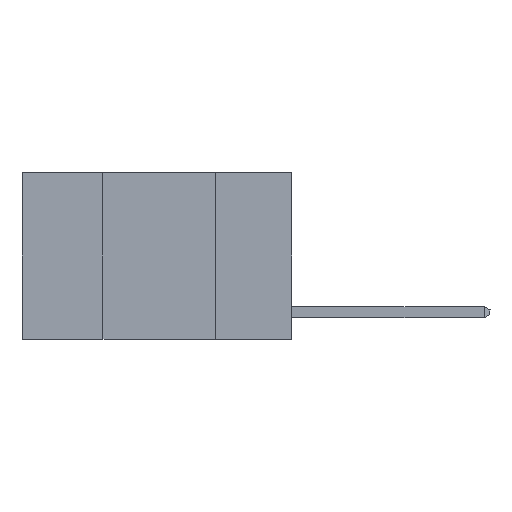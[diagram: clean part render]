
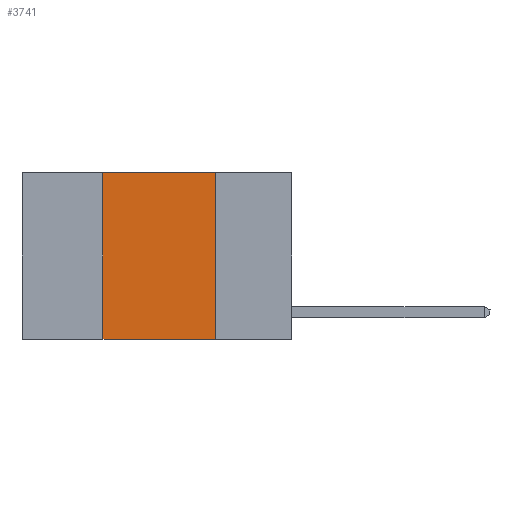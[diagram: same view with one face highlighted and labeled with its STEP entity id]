
A CAD part, left-side view. The second image highlights one B-rep face of the part: STEP entity #3741.
In plain terms, the highlighted planar face has unit normal (-1, 0, 0).
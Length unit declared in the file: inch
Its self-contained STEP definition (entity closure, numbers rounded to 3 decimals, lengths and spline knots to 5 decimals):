
#1185 = CARTESIAN_POINT ( 'NONE',  ( 0., 0.17, 0. ) ) ;
#2030 = ORIENTED_EDGE ( 'NONE', *, *, #6733, .F. ) ;
#2066 = LINE ( 'NONE', #9110, #14103 ) ;
#2395 = CARTESIAN_POINT ( 'NONE',  ( 0., 0.6, -0.37 ) ) ;
#2451 = DIRECTION ( 'NONE',  ( 0., 0., 1. ) ) ;
#3520 = PLANE ( 'NONE',  #16360 ) ;
#3563 = EDGE_CURVE ( 'NONE', #4761, #16960, #13905, .T. ) ;
#3741 = ADVANCED_FACE ( 'NONE', ( #8626 ), #3520, .F. ) ;
#4301 = ORIENTED_EDGE ( 'NONE', *, *, #13731, .F. ) ;
#4694 = CARTESIAN_POINT ( 'NONE',  ( 0., 0.6, 0. ) ) ;
#4761 = VERTEX_POINT ( 'NONE', #1185 ) ;
#5012 = LINE ( 'NONE', #2395, #15634 ) ;
#6733 = EDGE_CURVE ( 'NONE', #12757, #4761, #2066, .T. ) ;
#7668 = CARTESIAN_POINT ( 'NONE',  ( 0., 0.42, 0. ) ) ;
#8274 = DIRECTION ( 'NONE',  ( 0., 0., -1. ) ) ;
#8545 = VECTOR ( 'NONE', #2451, 39.37008 ) ;
#8626 = FACE_OUTER_BOUND ( 'NONE', #15045, .T. ) ;
#8893 = DIRECTION ( 'NONE',  ( 1., 0., 0. ) ) ;
#8979 = LINE ( 'NONE', #7668, #8545 ) ;
#9110 = CARTESIAN_POINT ( 'NONE',  ( 0., 0.6, 0. ) ) ;
#9703 = EDGE_CURVE ( 'NONE', #14587, #16960, #5012, .T. ) ;
#10130 = DIRECTION ( 'NONE',  ( 0., 0., -1. ) ) ;
#11974 = DIRECTION ( 'NONE',  ( 0., -1., 0. ) ) ;
#12148 = ORIENTED_EDGE ( 'NONE', *, *, #3563, .F. ) ;
#12649 = CARTESIAN_POINT ( 'NONE',  ( 0., 0.17, 0. ) ) ;
#12757 = VERTEX_POINT ( 'NONE', #13149 ) ;
#13138 = ORIENTED_EDGE ( 'NONE', *, *, #9703, .T. ) ;
#13149 = CARTESIAN_POINT ( 'NONE',  ( 0., 0.42, 0. ) ) ;
#13731 = EDGE_CURVE ( 'NONE', #14587, #12757, #8979, .T. ) ;
#13905 = LINE ( 'NONE', #12649, #15800 ) ;
#14103 = VECTOR ( 'NONE', #11974, 39.37008 ) ;
#14587 = VERTEX_POINT ( 'NONE', #14819 ) ;
#14632 = CARTESIAN_POINT ( 'NONE',  ( 0., 0.17, -0.37 ) ) ;
#14819 = CARTESIAN_POINT ( 'NONE',  ( 0., 0.42, -0.37 ) ) ;
#15045 = EDGE_LOOP ( 'NONE', ( #12148, #2030, #4301, #13138 ) ) ;
#15634 = VECTOR ( 'NONE', #17519, 39.37008 ) ;
#15800 = VECTOR ( 'NONE', #8274, 39.37008 ) ;
#16360 = AXIS2_PLACEMENT_3D ( 'NONE', #4694, #8893, #10130 ) ;
#16960 = VERTEX_POINT ( 'NONE', #14632 ) ;
#17519 = DIRECTION ( 'NONE',  ( 0., -1., 0. ) ) ;
